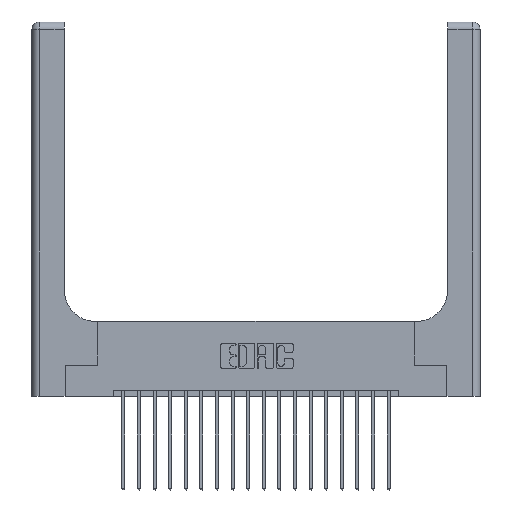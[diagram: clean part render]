
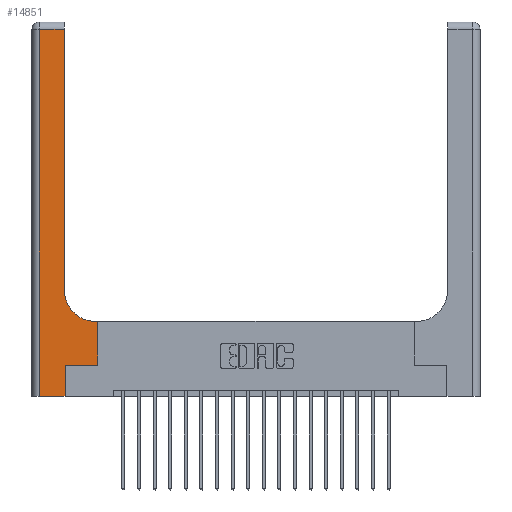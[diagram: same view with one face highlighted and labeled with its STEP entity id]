
A CAD part, top view. The second image highlights one B-rep face of the part: STEP entity #14851.
In plain terms, the highlighted planar face has unit normal (0, 0, 1).
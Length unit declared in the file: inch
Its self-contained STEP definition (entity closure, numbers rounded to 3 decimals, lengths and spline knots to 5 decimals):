
#13 = DIRECTION ( 'NONE',  ( 0., 0., -1. ) ) ;
#132 = VECTOR ( 'NONE', #17130, 39.37008 ) ;
#379 = CARTESIAN_POINT ( 'NONE',  ( 0.528, 0.25, 0.37 ) ) ;
#401 = LINE ( 'NONE', #2847, #14470 ) ;
#410 = EDGE_CURVE ( 'NONE', #3428, #9060, #8859, .T. ) ;
#597 = AXIS2_PLACEMENT_3D ( 'NONE', #15510, #13, #6373 ) ;
#645 = ORIENTED_EDGE ( 'NONE', *, *, #6424, .T. ) ;
#686 = VERTEX_POINT ( 'NONE', #16266 ) ;
#964 = VECTOR ( 'NONE', #6692, 39.37008 ) ;
#1019 = CARTESIAN_POINT ( 'NONE',  ( 0.265, 0., 0.37 ) ) ;
#2028 = CARTESIAN_POINT ( 'NONE',  ( 0., 0., 0.37 ) ) ;
#2687 = ORIENTED_EDGE ( 'NONE', *, *, #9640, .T. ) ;
#2847 = CARTESIAN_POINT ( 'NONE',  ( 0.06, 3., 0.37 ) ) ;
#3428 = VERTEX_POINT ( 'NONE', #11557 ) ;
#4134 = AXIS2_PLACEMENT_3D ( 'NONE', #4159, #15038, #8929 ) ;
#4159 = CARTESIAN_POINT ( 'NONE',  ( 0.51, 0.85, 0.37 ) ) ;
#4282 = EDGE_CURVE ( 'NONE', #6819, #686, #19471, .T. ) ;
#5237 = ORIENTED_EDGE ( 'NONE', *, *, #410, .T. ) ;
#5867 = DIRECTION ( 'NONE',  ( -1., 0., 0. ) ) ;
#6373 = DIRECTION ( 'NONE',  ( -1., 0., 0. ) ) ;
#6424 = EDGE_CURVE ( 'NONE', #686, #7474, #401, .T. ) ;
#6692 = DIRECTION ( 'NONE',  ( 1., 0., 0. ) ) ;
#6819 = VERTEX_POINT ( 'NONE', #17082 ) ;
#7010 = LINE ( 'NONE', #12490, #10406 ) ;
#7092 = ORIENTED_EDGE ( 'NONE', *, *, #15237, .T. ) ;
#7297 = CARTESIAN_POINT ( 'NONE',  ( 0., 2.94, 0.37 ) ) ;
#7474 = VERTEX_POINT ( 'NONE', #9735 ) ;
#7942 = ORIENTED_EDGE ( 'NONE', *, *, #13617, .T. ) ;
#8074 = EDGE_LOOP ( 'NONE', ( #16781, #11746, #645, #12039, #7942, #19991, #2687, #5237, #7092 ) ) ;
#8829 = CARTESIAN_POINT ( 'NONE',  ( 0.51, 0.6, 0.37 ) ) ;
#8859 = LINE ( 'NONE', #9147, #132 ) ;
#8929 = DIRECTION ( 'NONE',  ( 1., 0., 0. ) ) ;
#9060 = VERTEX_POINT ( 'NONE', #8829 ) ;
#9147 = CARTESIAN_POINT ( 'NONE',  ( 0.26, 0.6, 0.37 ) ) ;
#9284 = VECTOR ( 'NONE', #12078, 39.37008 ) ;
#9318 = PLANE ( 'NONE',  #597 ) ;
#9640 = EDGE_CURVE ( 'NONE', #9756, #3428, #19072, .T. ) ;
#9735 = CARTESIAN_POINT ( 'NONE',  ( 0.06, 0., 0.37 ) ) ;
#9756 = VERTEX_POINT ( 'NONE', #19585 ) ;
#10406 = VECTOR ( 'NONE', #17226, 39.37008 ) ;
#10675 = LINE ( 'NONE', #2028, #964 ) ;
#11019 = LINE ( 'NONE', #18175, #19597 ) ;
#11407 = DIRECTION ( 'NONE',  ( 0., 1., 0. ) ) ;
#11418 = LINE ( 'NONE', #15301, #9284 ) ;
#11557 = CARTESIAN_POINT ( 'NONE',  ( 0.528, 0.6, 0.37 ) ) ;
#11699 = VECTOR ( 'NONE', #11407, 39.37008 ) ;
#11736 = EDGE_CURVE ( 'NONE', #7474, #18613, #10675, .T. ) ;
#11746 = ORIENTED_EDGE ( 'NONE', *, *, #4282, .T. ) ;
#12039 = ORIENTED_EDGE ( 'NONE', *, *, #11736, .T. ) ;
#12078 = DIRECTION ( 'NONE',  ( 0., 1., 0. ) ) ;
#12380 = CARTESIAN_POINT ( 'NONE',  ( 0.265, 0.25, 0.37 ) ) ;
#12490 = CARTESIAN_POINT ( 'NONE',  ( 0.265, 0.25, 0.37 ) ) ;
#13617 = EDGE_CURVE ( 'NONE', #18613, #19536, #11418, .T. ) ;
#14470 = VECTOR ( 'NONE', #15100, 39.37008 ) ;
#14673 = VERTEX_POINT ( 'NONE', #16465 ) ;
#14851 = ADVANCED_FACE ( 'NONE', ( #15550 ), #9318, .F. ) ;
#14866 = EDGE_CURVE ( 'NONE', #19536, #9756, #7010, .T. ) ;
#14992 = DIRECTION ( 'NONE',  ( 0., 1., 0. ) ) ;
#15038 = DIRECTION ( 'NONE',  ( 0., 0., -1. ) ) ;
#15100 = DIRECTION ( 'NONE',  ( 0., -1., 0. ) ) ;
#15237 = EDGE_CURVE ( 'NONE', #9060, #14673, #17490, .T. ) ;
#15301 = CARTESIAN_POINT ( 'NONE',  ( 0.265, 0., 0.37 ) ) ;
#15510 = CARTESIAN_POINT ( 'NONE',  ( 0., 3., 0.37 ) ) ;
#15550 = FACE_OUTER_BOUND ( 'NONE', #8074, .T. ) ;
#16266 = CARTESIAN_POINT ( 'NONE',  ( 0.06, 2.94, 0.37 ) ) ;
#16465 = CARTESIAN_POINT ( 'NONE',  ( 0.26, 0.85, 0.37 ) ) ;
#16781 = ORIENTED_EDGE ( 'NONE', *, *, #18600, .T. ) ;
#17082 = CARTESIAN_POINT ( 'NONE',  ( 0.26, 2.94, 0.37 ) ) ;
#17130 = DIRECTION ( 'NONE',  ( -1., 0., 0. ) ) ;
#17226 = DIRECTION ( 'NONE',  ( 1., 0., 0. ) ) ;
#17490 = CIRCLE ( 'NONE', #4134, 0.25 ) ;
#18175 = CARTESIAN_POINT ( 'NONE',  ( 0.26, 3., 0.37 ) ) ;
#18270 = VECTOR ( 'NONE', #5867, 39.37008 ) ;
#18600 = EDGE_CURVE ( 'NONE', #14673, #6819, #11019, .T. ) ;
#18613 = VERTEX_POINT ( 'NONE', #1019 ) ;
#19072 = LINE ( 'NONE', #379, #11699 ) ;
#19471 = LINE ( 'NONE', #7297, #18270 ) ;
#19536 = VERTEX_POINT ( 'NONE', #12380 ) ;
#19585 = CARTESIAN_POINT ( 'NONE',  ( 0.528, 0.25, 0.37 ) ) ;
#19597 = VECTOR ( 'NONE', #14992, 39.37008 ) ;
#19991 = ORIENTED_EDGE ( 'NONE', *, *, #14866, .T. ) ;
